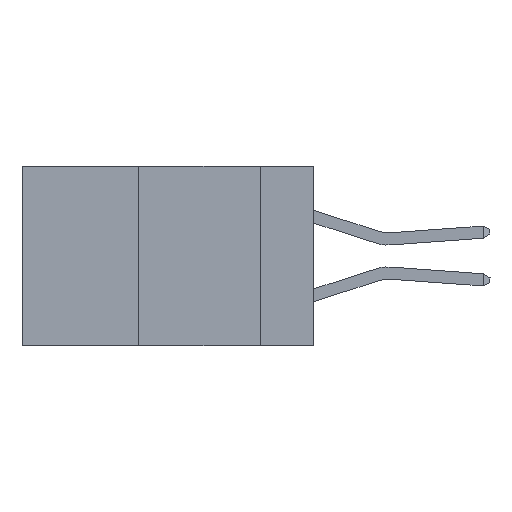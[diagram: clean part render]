
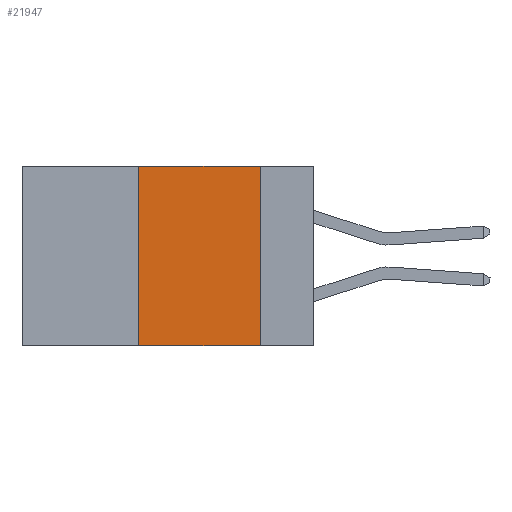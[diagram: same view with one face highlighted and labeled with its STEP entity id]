
A CAD part, left-side view. The second image highlights one B-rep face of the part: STEP entity #21947.
In plain terms, the highlighted planar face has unit normal (-1, 0, 0).
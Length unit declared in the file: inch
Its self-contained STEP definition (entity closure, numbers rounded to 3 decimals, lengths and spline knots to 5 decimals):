
#184 = LINE ( 'NONE', #17248, #4332 ) ;
#1452 = VERTEX_POINT ( 'NONE', #4284 ) ;
#2721 = DIRECTION ( 'NONE',  ( 0., -1., 0. ) ) ;
#3369 = ORIENTED_EDGE ( 'NONE', *, *, #30631, .F. ) ;
#4284 = CARTESIAN_POINT ( 'NONE',  ( 0., 0.36, -0.37 ) ) ;
#4332 = VECTOR ( 'NONE', #15064, 39.37008 ) ;
#5160 = VECTOR ( 'NONE', #6228, 39.37008 ) ;
#6217 = ORIENTED_EDGE ( 'NONE', *, *, #22654, .F. ) ;
#6228 = DIRECTION ( 'NONE',  ( 0., -1., 0. ) ) ;
#6375 = LINE ( 'NONE', #31567, #5160 ) ;
#7869 = EDGE_CURVE ( 'NONE', #15343, #22434, #6375, .T. ) ;
#8157 = FACE_OUTER_BOUND ( 'NONE', #10778, .T. ) ;
#9313 = VERTEX_POINT ( 'NONE', #13103 ) ;
#10778 = EDGE_LOOP ( 'NONE', ( #6217, #14908, #3369, #28729 ) ) ;
#12273 = PLANE ( 'NONE',  #25591 ) ;
#13103 = CARTESIAN_POINT ( 'NONE',  ( 0., 0.11, -0.37 ) ) ;
#14908 = ORIENTED_EDGE ( 'NONE', *, *, #7869, .F. ) ;
#15064 = DIRECTION ( 'NONE',  ( 0., 0., 1. ) ) ;
#15239 = DIRECTION ( 'NONE',  ( 1., 0., 0. ) ) ;
#15343 = VERTEX_POINT ( 'NONE', #22677 ) ;
#17248 = CARTESIAN_POINT ( 'NONE',  ( 0., 0.36, 0. ) ) ;
#17480 = VECTOR ( 'NONE', #31339, 39.37008 ) ;
#17647 = CARTESIAN_POINT ( 'NONE',  ( 0., 0.6, 0. ) ) ;
#18360 = LINE ( 'NONE', #33801, #24489 ) ;
#21361 = EDGE_CURVE ( 'NONE', #1452, #9313, #18360, .T. ) ;
#21947 = ADVANCED_FACE ( 'NONE', ( #8157 ), #12273, .F. ) ;
#22434 = VERTEX_POINT ( 'NONE', #24820 ) ;
#22654 = EDGE_CURVE ( 'NONE', #22434, #9313, #25277, .T. ) ;
#22677 = CARTESIAN_POINT ( 'NONE',  ( 0., 0.36, 0. ) ) ;
#24489 = VECTOR ( 'NONE', #2721, 39.37008 ) ;
#24820 = CARTESIAN_POINT ( 'NONE',  ( 0., 0.11, 0. ) ) ;
#25277 = LINE ( 'NONE', #28695, #17480 ) ;
#25591 = AXIS2_PLACEMENT_3D ( 'NONE', #17647, #15239, #25751 ) ;
#25751 = DIRECTION ( 'NONE',  ( 0., 0., -1. ) ) ;
#28695 = CARTESIAN_POINT ( 'NONE',  ( 0., 0.11, 0. ) ) ;
#28729 = ORIENTED_EDGE ( 'NONE', *, *, #21361, .T. ) ;
#30631 = EDGE_CURVE ( 'NONE', #1452, #15343, #184, .T. ) ;
#31339 = DIRECTION ( 'NONE',  ( 0., 0., -1. ) ) ;
#31567 = CARTESIAN_POINT ( 'NONE',  ( 0., 0.6, 0. ) ) ;
#33801 = CARTESIAN_POINT ( 'NONE',  ( 0., 0.6, -0.37 ) ) ;
